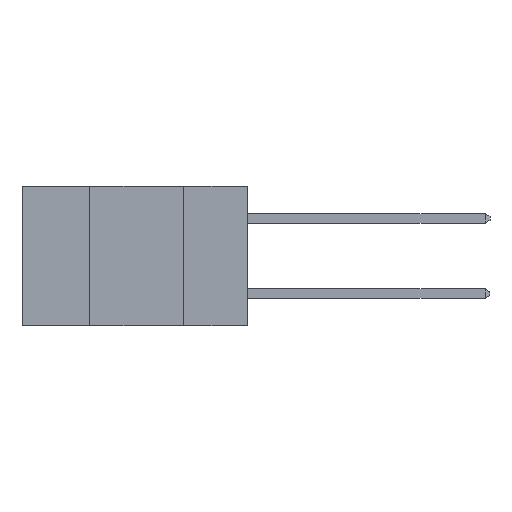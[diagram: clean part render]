
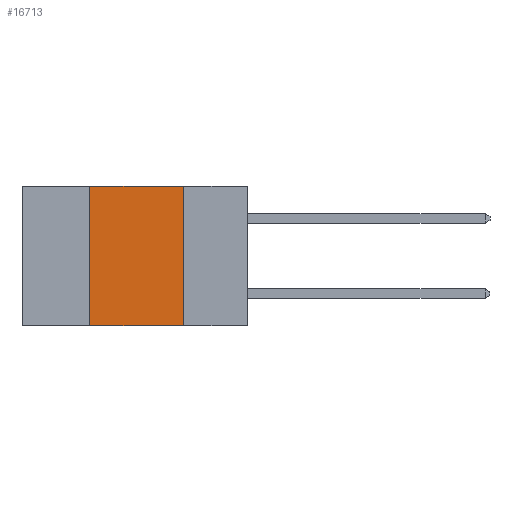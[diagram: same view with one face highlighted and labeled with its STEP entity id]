
A CAD part, left-side view. The second image highlights one B-rep face of the part: STEP entity #16713.
In plain terms, the highlighted planar face has unit normal (-1, 0, 0).
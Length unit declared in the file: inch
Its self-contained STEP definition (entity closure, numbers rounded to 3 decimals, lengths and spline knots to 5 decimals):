
#134 = CARTESIAN_POINT ( 'NONE',  ( 0., 0.6, 0. ) ) ;
#1316 = VECTOR ( 'NONE', #4084, 39.37008 ) ;
#1909 = LINE ( 'NONE', #5204, #19752 ) ;
#2625 = VECTOR ( 'NONE', #17210, 39.37008 ) ;
#4084 = DIRECTION ( 'NONE',  ( 0., 0., 1. ) ) ;
#4111 = LINE ( 'NONE', #5632, #2625 ) ;
#5204 = CARTESIAN_POINT ( 'NONE',  ( 0., 0.6, 0. ) ) ;
#5632 = CARTESIAN_POINT ( 'NONE',  ( 0., 0.17, 0. ) ) ;
#5882 = EDGE_CURVE ( 'NONE', #13077, #29257, #15306, .T. ) ;
#9022 = ORIENTED_EDGE ( 'NONE', *, *, #9612, .T. ) ;
#9331 = CARTESIAN_POINT ( 'NONE',  ( 0., 0.17, 0. ) ) ;
#9612 = EDGE_CURVE ( 'NONE', #13077, #10036, #15516, .T. ) ;
#10036 = VERTEX_POINT ( 'NONE', #18646 ) ;
#10142 = VECTOR ( 'NONE', #21257, 39.37008 ) ;
#10991 = ORIENTED_EDGE ( 'NONE', *, *, #5882, .F. ) ;
#11987 = CARTESIAN_POINT ( 'NONE',  ( 0., 0.42, -0.37 ) ) ;
#12093 = DIRECTION ( 'NONE',  ( 0., 0., -1. ) ) ;
#13077 = VERTEX_POINT ( 'NONE', #11987 ) ;
#13363 = ORIENTED_EDGE ( 'NONE', *, *, #18014, .F. ) ;
#14409 = CARTESIAN_POINT ( 'NONE',  ( 0., 0.6, -0.37 ) ) ;
#14631 = DIRECTION ( 'NONE',  ( 0., -1., 0. ) ) ;
#15306 = LINE ( 'NONE', #22605, #1316 ) ;
#15516 = LINE ( 'NONE', #14409, #10142 ) ;
#16654 = ORIENTED_EDGE ( 'NONE', *, *, #18875, .F. ) ;
#16713 = ADVANCED_FACE ( 'NONE', ( #18777 ), #21148, .F. ) ;
#17210 = DIRECTION ( 'NONE',  ( 0., 0., -1. ) ) ;
#18014 = EDGE_CURVE ( 'NONE', #29257, #27165, #1909, .T. ) ;
#18646 = CARTESIAN_POINT ( 'NONE',  ( 0., 0.17, -0.37 ) ) ;
#18777 = FACE_OUTER_BOUND ( 'NONE', #21076, .T. ) ;
#18875 = EDGE_CURVE ( 'NONE', #27165, #10036, #4111, .T. ) ;
#19752 = VECTOR ( 'NONE', #14631, 39.37008 ) ;
#20104 = AXIS2_PLACEMENT_3D ( 'NONE', #134, #25707, #12093 ) ;
#21076 = EDGE_LOOP ( 'NONE', ( #16654, #13363, #10991, #9022 ) ) ;
#21148 = PLANE ( 'NONE',  #20104 ) ;
#21176 = CARTESIAN_POINT ( 'NONE',  ( 0., 0.42, 0. ) ) ;
#21257 = DIRECTION ( 'NONE',  ( 0., -1., 0. ) ) ;
#22605 = CARTESIAN_POINT ( 'NONE',  ( 0., 0.42, 0. ) ) ;
#25707 = DIRECTION ( 'NONE',  ( 1., 0., 0. ) ) ;
#27165 = VERTEX_POINT ( 'NONE', #9331 ) ;
#29257 = VERTEX_POINT ( 'NONE', #21176 ) ;
